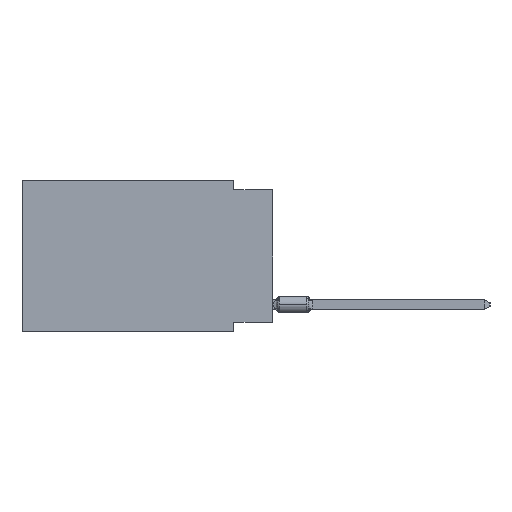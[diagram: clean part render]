
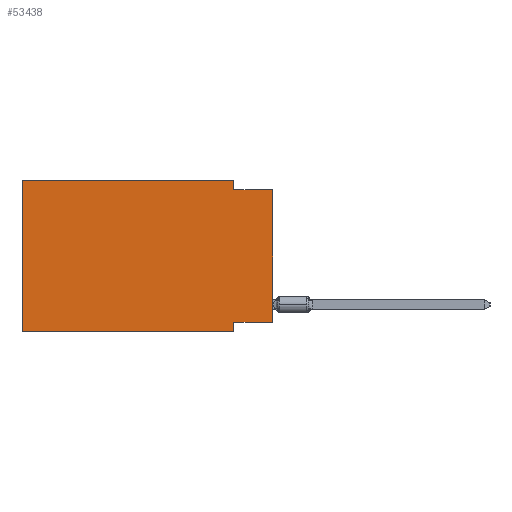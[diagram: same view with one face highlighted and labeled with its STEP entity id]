
A CAD part, left-side view. The second image highlights one B-rep face of the part: STEP entity #53438.
In plain terms, the highlighted planar face has unit normal (-1, 0, 0).
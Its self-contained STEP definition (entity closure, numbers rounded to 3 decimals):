
#1646 = EDGE_CURVE ( 'NONE', #24543, #10008, #54028, .T. ) ;
#1930 = CARTESIAN_POINT ( 'NONE',  ( 0., 2.54, -9.271 ) ) ;
#3457 = ORIENTED_EDGE ( 'NONE', *, *, #50754, .F. ) ;
#4517 = CARTESIAN_POINT ( 'NONE',  ( 0., 16.383, -9.906 ) ) ;
#4825 = DIRECTION ( 'NONE',  ( 0., 0., -1. ) ) ;
#6025 = PLANE ( 'NONE',  #35917 ) ;
#6372 = CARTESIAN_POINT ( 'NONE',  ( 0., 2.54, 0. ) ) ;
#8390 = VERTEX_POINT ( 'NONE', #36514 ) ;
#9353 = CARTESIAN_POINT ( 'NONE',  ( 0., 0., 0. ) ) ;
#9610 = ORIENTED_EDGE ( 'NONE', *, *, #32731, .F. ) ;
#10008 = VERTEX_POINT ( 'NONE', #58137 ) ;
#10129 = VERTEX_POINT ( 'NONE', #1930 ) ;
#11393 = EDGE_CURVE ( 'NONE', #10129, #10008, #54331, .T. ) ;
#11490 = CARTESIAN_POINT ( 'NONE',  ( 0., 0., -9.271 ) ) ;
#12124 = VECTOR ( 'NONE', #62568, 1000. ) ;
#12917 = DIRECTION ( 'NONE',  ( 0., 0., 1. ) ) ;
#17226 = DIRECTION ( 'NONE',  ( 0., 1., 0. ) ) ;
#19562 = DIRECTION ( 'NONE',  ( 0., 0., -1. ) ) ;
#19681 = VERTEX_POINT ( 'NONE', #23250 ) ;
#20780 = CARTESIAN_POINT ( 'NONE',  ( 0., 16.383, 0. ) ) ;
#20820 = VECTOR ( 'NONE', #12917, 1000. ) ;
#21736 = VECTOR ( 'NONE', #29673, 1000. ) ;
#21897 = CARTESIAN_POINT ( 'NONE',  ( 0., 0., -0.635 ) ) ;
#23250 = CARTESIAN_POINT ( 'NONE',  ( 0., 2.54, -0.635 ) ) ;
#23387 = CARTESIAN_POINT ( 'NONE',  ( 0., 16.383, 0. ) ) ;
#24149 = VERTEX_POINT ( 'NONE', #11490 ) ;
#24543 = VERTEX_POINT ( 'NONE', #30121 ) ;
#24807 = CARTESIAN_POINT ( 'NONE',  ( 0., 2.54, -9.906 ) ) ;
#24811 = DIRECTION ( 'NONE',  ( 1., 0., 0. ) ) ;
#24828 = DIRECTION ( 'NONE',  ( 0., -1., 0. ) ) ;
#25875 = ORIENTED_EDGE ( 'NONE', *, *, #34091, .F. ) ;
#26741 = LINE ( 'NONE', #61822, #60646 ) ;
#27667 = CARTESIAN_POINT ( 'NONE',  ( 0., 16.383, 0. ) ) ;
#27942 = ORIENTED_EDGE ( 'NONE', *, *, #1646, .T. ) ;
#29673 = DIRECTION ( 'NONE',  ( 0., 0., -1. ) ) ;
#29742 = FACE_OUTER_BOUND ( 'NONE', #42859, .T. ) ;
#30121 = CARTESIAN_POINT ( 'NONE',  ( 0., 16.383, -9.906 ) ) ;
#32731 = EDGE_CURVE ( 'NONE', #47777, #19681, #44446, .T. ) ;
#32991 = LINE ( 'NONE', #9353, #60591 ) ;
#34091 = EDGE_CURVE ( 'NONE', #24543, #8390, #57827, .T. ) ;
#34564 = EDGE_CURVE ( 'NONE', #24149, #10129, #26741, .T. ) ;
#35917 = AXIS2_PLACEMENT_3D ( 'NONE', #20780, #24811, #4825 ) ;
#36084 = EDGE_CURVE ( 'NONE', #24149, #60336, #32991, .T. ) ;
#36514 = CARTESIAN_POINT ( 'NONE',  ( 0., 16.383, 0. ) ) ;
#38482 = DIRECTION ( 'NONE',  ( 0., -1., 0. ) ) ;
#42739 = EDGE_CURVE ( 'NONE', #8390, #47777, #43414, .T. ) ;
#42859 = EDGE_LOOP ( 'NONE', ( #52443, #3457, #9610, #56024, #25875, #27942, #58946, #54354 ) ) ;
#43414 = LINE ( 'NONE', #23387, #48217 ) ;
#44116 = CARTESIAN_POINT ( 'NONE',  ( 0., 2.54, 0. ) ) ;
#44446 = LINE ( 'NONE', #44116, #21736 ) ;
#47501 = CARTESIAN_POINT ( 'NONE',  ( 0., 0., -0.635 ) ) ;
#47777 = VERTEX_POINT ( 'NONE', #6372 ) ;
#48217 = VECTOR ( 'NONE', #38482, 1000. ) ;
#48371 = DIRECTION ( 'NONE',  ( 0., 0., 1. ) ) ;
#50754 = EDGE_CURVE ( 'NONE', #19681, #60336, #52738, .T. ) ;
#52443 = ORIENTED_EDGE ( 'NONE', *, *, #36084, .T. ) ;
#52738 = LINE ( 'NONE', #47501, #12124 ) ;
#53347 = VECTOR ( 'NONE', #19562, 1000. ) ;
#53438 = ADVANCED_FACE ( 'NONE', ( #29742 ), #6025, .F. ) ;
#54028 = LINE ( 'NONE', #4517, #55684 ) ;
#54331 = LINE ( 'NONE', #24807, #53347 ) ;
#54354 = ORIENTED_EDGE ( 'NONE', *, *, #34564, .F. ) ;
#55684 = VECTOR ( 'NONE', #24828, 1000. ) ;
#56024 = ORIENTED_EDGE ( 'NONE', *, *, #42739, .F. ) ;
#57827 = LINE ( 'NONE', #27667, #20820 ) ;
#58137 = CARTESIAN_POINT ( 'NONE',  ( 0., 2.54, -9.906 ) ) ;
#58946 = ORIENTED_EDGE ( 'NONE', *, *, #11393, .F. ) ;
#60336 = VERTEX_POINT ( 'NONE', #21897 ) ;
#60591 = VECTOR ( 'NONE', #48371, 1000. ) ;
#60646 = VECTOR ( 'NONE', #17226, 1000. ) ;
#61822 = CARTESIAN_POINT ( 'NONE',  ( 0., 0., -9.271 ) ) ;
#62568 = DIRECTION ( 'NONE',  ( 0., -1., 0. ) ) ;
